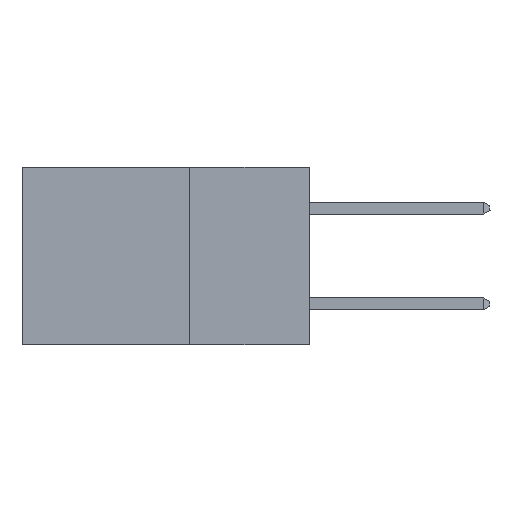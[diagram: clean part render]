
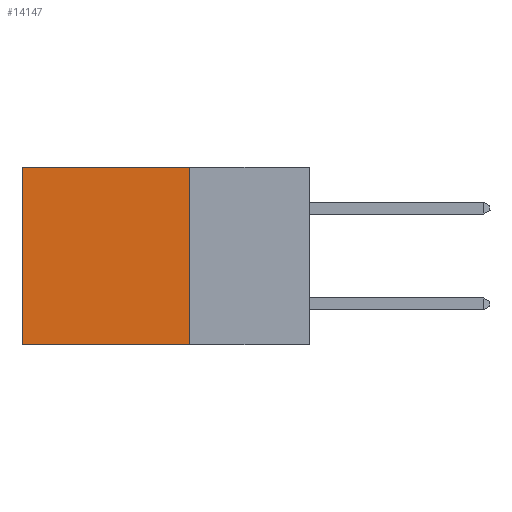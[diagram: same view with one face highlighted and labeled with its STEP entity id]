
A CAD part, left-side view. The second image highlights one B-rep face of the part: STEP entity #14147.
In plain terms, the highlighted planar face has unit normal (-1, 0, 0).
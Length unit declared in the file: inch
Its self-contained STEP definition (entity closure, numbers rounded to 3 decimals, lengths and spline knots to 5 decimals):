
#498 = VECTOR ( 'NONE', #7039, 39.37008 ) ;
#835 = EDGE_CURVE ( 'NONE', #25238, #24631, #17403, .T. ) ;
#1545 = EDGE_CURVE ( 'NONE', #13399, #22999, #22812, .T. ) ;
#1606 = PLANE ( 'NONE',  #16939 ) ;
#1610 = CARTESIAN_POINT ( 'NONE',  ( 0.2875, 0.25, 0. ) ) ;
#2725 = EDGE_LOOP ( 'NONE', ( #6299, #17794, #24638, #15345 ) ) ;
#3997 = CARTESIAN_POINT ( 'NONE',  ( 0.2875, 0.25, -0.37 ) ) ;
#6071 = LINE ( 'NONE', #16415, #18567 ) ;
#6299 = ORIENTED_EDGE ( 'NONE', *, *, #25150, .T. ) ;
#7039 = DIRECTION ( 'NONE',  ( 0., 1., 0. ) ) ;
#7841 = FACE_OUTER_BOUND ( 'NONE', #2725, .T. ) ;
#8315 = VECTOR ( 'NONE', #14594, 39.37008 ) ;
#8708 = CARTESIAN_POINT ( 'NONE',  ( 0.2875, 0.25, -0.37 ) ) ;
#9335 = CARTESIAN_POINT ( 'NONE',  ( 0.2875, 0.25, 0. ) ) ;
#11917 = DIRECTION ( 'NONE',  ( 0., 0., -1. ) ) ;
#12170 = DIRECTION ( 'NONE',  ( 0., 0., -1. ) ) ;
#13399 = VERTEX_POINT ( 'NONE', #8708 ) ;
#14147 = ADVANCED_FACE ( 'NONE', ( #7841 ), #1606, .F. ) ;
#14388 = VECTOR ( 'NONE', #24108, 39.37008 ) ;
#14594 = DIRECTION ( 'NONE',  ( 0., 1., 0. ) ) ;
#15345 = ORIENTED_EDGE ( 'NONE', *, *, #835, .T. ) ;
#15589 = EDGE_CURVE ( 'NONE', #25238, #13399, #20288, .T. ) ;
#16249 = CARTESIAN_POINT ( 'NONE',  ( 0.2875, 0.6, -0.37 ) ) ;
#16415 = CARTESIAN_POINT ( 'NONE',  ( 0.2875, 0.6, 0. ) ) ;
#16939 = AXIS2_PLACEMENT_3D ( 'NONE', #18234, #18365, #11917 ) ;
#17403 = LINE ( 'NONE', #9335, #498 ) ;
#17794 = ORIENTED_EDGE ( 'NONE', *, *, #1545, .F. ) ;
#18234 = CARTESIAN_POINT ( 'NONE',  ( 0.2875, 0.25, 0. ) ) ;
#18276 = CARTESIAN_POINT ( 'NONE',  ( 0.2875, 0.6, 0. ) ) ;
#18365 = DIRECTION ( 'NONE',  ( 1., 0., 0. ) ) ;
#18567 = VECTOR ( 'NONE', #12170, 39.37008 ) ;
#19600 = CARTESIAN_POINT ( 'NONE',  ( 0.2875, 0.25, 0. ) ) ;
#20288 = LINE ( 'NONE', #1610, #14388 ) ;
#22812 = LINE ( 'NONE', #3997, #8315 ) ;
#22999 = VERTEX_POINT ( 'NONE', #16249 ) ;
#24108 = DIRECTION ( 'NONE',  ( 0., 0., -1. ) ) ;
#24631 = VERTEX_POINT ( 'NONE', #18276 ) ;
#24638 = ORIENTED_EDGE ( 'NONE', *, *, #15589, .F. ) ;
#25150 = EDGE_CURVE ( 'NONE', #24631, #22999, #6071, .T. ) ;
#25238 = VERTEX_POINT ( 'NONE', #19600 ) ;
